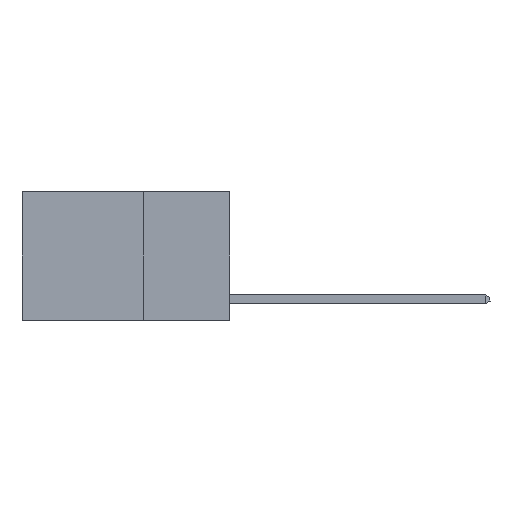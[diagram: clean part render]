
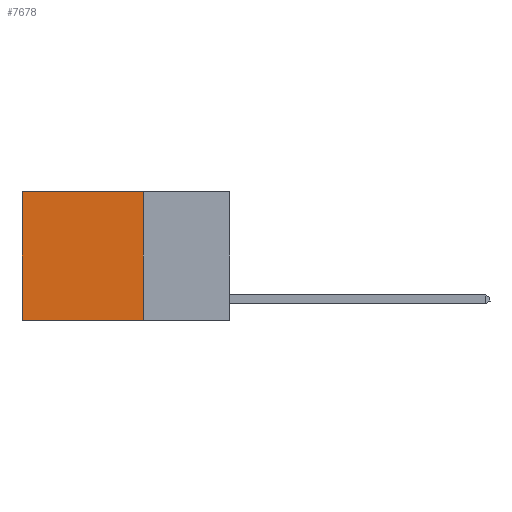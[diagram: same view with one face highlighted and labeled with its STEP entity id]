
A CAD part, left-side view. The second image highlights one B-rep face of the part: STEP entity #7678.
In plain terms, the highlighted planar face has unit normal (-1, 0, 0).
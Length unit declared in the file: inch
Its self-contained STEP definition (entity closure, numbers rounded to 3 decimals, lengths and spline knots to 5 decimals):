
#275 = CARTESIAN_POINT ( 'NONE',  ( 0.2625, 0.25, -0.37 ) ) ;
#288 = CARTESIAN_POINT ( 'NONE',  ( 0.2625, 0.6, 0. ) ) ;
#805 = LINE ( 'NONE', #11126, #11969 ) ;
#1154 = DIRECTION ( 'NONE',  ( 0., 0., -1. ) ) ;
#1780 = PLANE ( 'NONE',  #9282 ) ;
#2560 = VERTEX_POINT ( 'NONE', #3964 ) ;
#2661 = VECTOR ( 'NONE', #1154, 39.37008 ) ;
#3144 = VERTEX_POINT ( 'NONE', #7087 ) ;
#3754 = ORIENTED_EDGE ( 'NONE', *, *, #12222, .T. ) ;
#3964 = CARTESIAN_POINT ( 'NONE',  ( 0.2625, 0.25, 0. ) ) ;
#4011 = DIRECTION ( 'NONE',  ( 1., 0., 0. ) ) ;
#4507 = CARTESIAN_POINT ( 'NONE',  ( 0.2625, 0.6, 0. ) ) ;
#4611 = ORIENTED_EDGE ( 'NONE', *, *, #6118, .F. ) ;
#4733 = VECTOR ( 'NONE', #12999, 39.37008 ) ;
#4902 = FACE_OUTER_BOUND ( 'NONE', #9638, .T. ) ;
#5424 = LINE ( 'NONE', #4507, #4733 ) ;
#5914 = LINE ( 'NONE', #11668, #8801 ) ;
#6118 = EDGE_CURVE ( 'NONE', #10359, #3144, #805, .T. ) ;
#6382 = DIRECTION ( 'NONE',  ( 0., 1., 0. ) ) ;
#6664 = CARTESIAN_POINT ( 'NONE',  ( 0.2625, 0.25, 0. ) ) ;
#6859 = ORIENTED_EDGE ( 'NONE', *, *, #8468, .F. ) ;
#6951 = DIRECTION ( 'NONE',  ( 0., 1., 0. ) ) ;
#7087 = CARTESIAN_POINT ( 'NONE',  ( 0.2625, 0.6, -0.37 ) ) ;
#7678 = ADVANCED_FACE ( 'NONE', ( #4902 ), #1780, .F. ) ;
#8145 = ORIENTED_EDGE ( 'NONE', *, *, #8421, .T. ) ;
#8421 = EDGE_CURVE ( 'NONE', #2560, #12368, #5914, .T. ) ;
#8468 = EDGE_CURVE ( 'NONE', #2560, #10359, #10582, .T. ) ;
#8801 = VECTOR ( 'NONE', #6382, 39.37008 ) ;
#9282 = AXIS2_PLACEMENT_3D ( 'NONE', #9398, #4011, #11504 ) ;
#9398 = CARTESIAN_POINT ( 'NONE',  ( 0.2625, 0.25, 0. ) ) ;
#9638 = EDGE_LOOP ( 'NONE', ( #3754, #4611, #6859, #8145 ) ) ;
#10359 = VERTEX_POINT ( 'NONE', #275 ) ;
#10582 = LINE ( 'NONE', #6664, #2661 ) ;
#11126 = CARTESIAN_POINT ( 'NONE',  ( 0.2625, 0.25, -0.37 ) ) ;
#11504 = DIRECTION ( 'NONE',  ( 0., 0., -1. ) ) ;
#11668 = CARTESIAN_POINT ( 'NONE',  ( 0.2625, 0.25, 0. ) ) ;
#11969 = VECTOR ( 'NONE', #6951, 39.37008 ) ;
#12222 = EDGE_CURVE ( 'NONE', #12368, #3144, #5424, .T. ) ;
#12368 = VERTEX_POINT ( 'NONE', #288 ) ;
#12999 = DIRECTION ( 'NONE',  ( 0., 0., -1. ) ) ;
